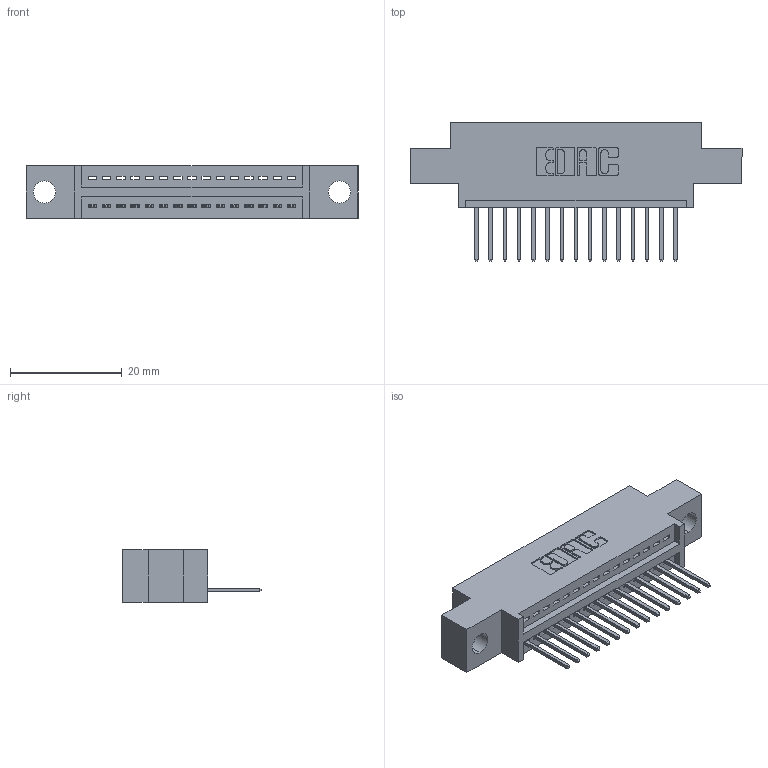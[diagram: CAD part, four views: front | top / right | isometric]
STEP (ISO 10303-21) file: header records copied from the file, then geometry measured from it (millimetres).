
FILE_DESCRIPTION (( 'STEP AP203' ), '1' );
FILE_NAME ('345-015-523-604.STEP', '2021-05-26T14:13:22', ( '' ), ( '' ), 'SwSTEP 2.0', 'SolidWorks 2020', '' );
FILE_SCHEMA (( 'CONFIG_CONTROL_DESIGN' ));
Length unit declared in the file: inch
Products named in the file (3): 345-015-523-604; 345-292-001_345-293-123; 345 Part_0.170 Offset - 0.156 Dia-TI
Assembly tree (16 placements, depth 2):
  345-015-523-604
    345 Part_0.170 Offset - 0.156 Dia-TI
    345-292-001_345-293-123  x15
Bounding box: 59.31 x 24.82 x 9.4 mm (x, y, z)
Volume: 5186.9 mm3; surface area: 6511.4 mm2
Topology: 16 solids, 16 shells, 1014 faces, 3029 edges, 1998 vertices
Faces by surface type: plane 698, cylinder 316
Entity records: 15493 total; most frequent: CARTESIAN_POINT 2695, ORIENTED_EDGE 2642, DIRECTION 2391, EDGE_CURVE 1321, LINE 1129, VECTOR 1129, VERTEX_POINT 878, AXIS2_PLACEMENT_3D 631
